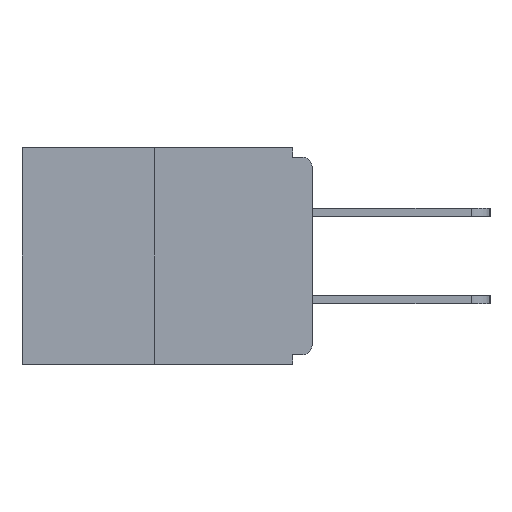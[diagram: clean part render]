
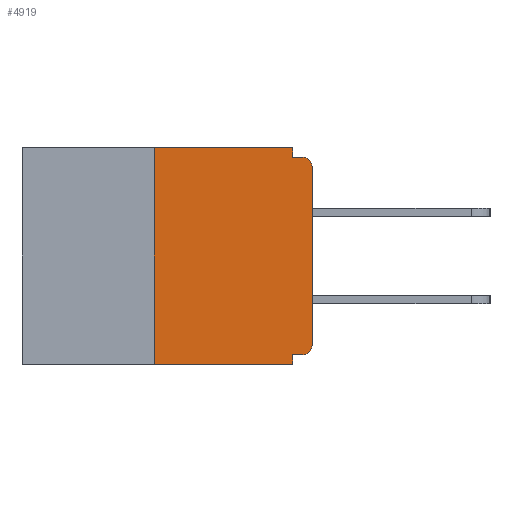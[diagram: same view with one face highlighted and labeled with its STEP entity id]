
A CAD part, left-side view. The second image highlights one B-rep face of the part: STEP entity #4919.
In plain terms, the highlighted planar face has unit normal (-1, 0, 0).
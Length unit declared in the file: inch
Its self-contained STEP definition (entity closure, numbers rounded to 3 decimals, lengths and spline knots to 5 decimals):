
#71 = DIRECTION ( 'NONE',  ( 0., 0., 1. ) ) ;
#465 = VECTOR ( 'NONE', #11201, 39.37008 ) ;
#682 = ORIENTED_EDGE ( 'NONE', *, *, #8445, .F. ) ;
#795 = EDGE_CURVE ( 'NONE', #11745, #6879, #1094, .T. ) ;
#845 = FACE_OUTER_BOUND ( 'NONE', #6350, .T. ) ;
#900 = CARTESIAN_POINT ( 'NONE',  ( 0., 0.25, 0. ) ) ;
#918 = CARTESIAN_POINT ( 'NONE',  ( 0., 0.031, -0.015 ) ) ;
#971 = CARTESIAN_POINT ( 'NONE',  ( 0., 0.25, 0. ) ) ;
#1028 = CARTESIAN_POINT ( 'NONE',  ( 0., 0.46, -0.343 ) ) ;
#1060 = CARTESIAN_POINT ( 'NONE',  ( 0., 0., -0.313 ) ) ;
#1094 = LINE ( 'NONE', #4861, #9689 ) ;
#1195 = EDGE_CURVE ( 'NONE', #1671, #11745, #11263, .T. ) ;
#1282 = AXIS2_PLACEMENT_3D ( 'NONE', #11019, #3575, #7242 ) ;
#1609 = LINE ( 'NONE', #9250, #11494 ) ;
#1671 = VERTEX_POINT ( 'NONE', #9463 ) ;
#1817 = CARTESIAN_POINT ( 'NONE',  ( 0., 0.46, 0. ) ) ;
#2178 = EDGE_CURVE ( 'NONE', #5679, #11479, #9388, .T. ) ;
#2274 = AXIS2_PLACEMENT_3D ( 'NONE', #6519, #6356, #4466 ) ;
#2526 = VERTEX_POINT ( 'NONE', #6142 ) ;
#2614 = VERTEX_POINT ( 'NONE', #918 ) ;
#2723 = ORIENTED_EDGE ( 'NONE', *, *, #6912, .T. ) ;
#2957 = ORIENTED_EDGE ( 'NONE', *, *, #3427, .F. ) ;
#3118 = DIRECTION ( 'NONE',  ( 0., -1., 0. ) ) ;
#3427 = EDGE_CURVE ( 'NONE', #11101, #5679, #6107, .T. ) ;
#3575 = DIRECTION ( 'NONE',  ( -1., 0., 0. ) ) ;
#3594 = ORIENTED_EDGE ( 'NONE', *, *, #4666, .T. ) ;
#3714 = DIRECTION ( 'NONE',  ( 0., 0., -1. ) ) ;
#3778 = VERTEX_POINT ( 'NONE', #9064 ) ;
#3984 = VECTOR ( 'NONE', #3118, 39.37008 ) ;
#4041 = LINE ( 'NONE', #1028, #3984 ) ;
#4174 = CARTESIAN_POINT ( 'NONE',  ( 0., 0.031, -0.343 ) ) ;
#4297 = CARTESIAN_POINT ( 'NONE',  ( 0., 0., -0.328 ) ) ;
#4466 = DIRECTION ( 'NONE',  ( 0., 0., -1. ) ) ;
#4479 = CIRCLE ( 'NONE', #2274, 0.015 ) ;
#4496 = EDGE_CURVE ( 'NONE', #2614, #2526, #9310, .T. ) ;
#4666 = EDGE_CURVE ( 'NONE', #10458, #3778, #7603, .T. ) ;
#4812 = VECTOR ( 'NONE', #8550, 39.37008 ) ;
#4861 = CARTESIAN_POINT ( 'NONE',  ( 0., 0.46, 0. ) ) ;
#4919 = ADVANCED_FACE ( 'NONE', ( #845 ), #8303, .F. ) ;
#4942 = ORIENTED_EDGE ( 'NONE', *, *, #2178, .F. ) ;
#5195 = DIRECTION ( 'NONE',  ( 0., 0., -1. ) ) ;
#5679 = VERTEX_POINT ( 'NONE', #11996 ) ;
#5929 = VECTOR ( 'NONE', #71, 39.37008 ) ;
#6107 = LINE ( 'NONE', #4297, #9466 ) ;
#6142 = CARTESIAN_POINT ( 'NONE',  ( 0., 0.015, -0.015 ) ) ;
#6230 = EDGE_CURVE ( 'NONE', #1671, #11479, #4041, .T. ) ;
#6350 = EDGE_LOOP ( 'NONE', ( #6984, #10186, #9036, #4942, #2957, #7260, #3594, #2723, #8424, #682 ) ) ;
#6356 = DIRECTION ( 'NONE',  ( -1., 0., 0. ) ) ;
#6420 = DIRECTION ( 'NONE',  ( 1., 0., 0. ) ) ;
#6519 = CARTESIAN_POINT ( 'NONE',  ( 0., 0.015, -0.03 ) ) ;
#6621 = CIRCLE ( 'NONE', #1282, 0.015 ) ;
#6879 = VERTEX_POINT ( 'NONE', #9213 ) ;
#6912 = EDGE_CURVE ( 'NONE', #3778, #2526, #4479, .T. ) ;
#6984 = ORIENTED_EDGE ( 'NONE', *, *, #795, .F. ) ;
#7242 = DIRECTION ( 'NONE',  ( 0., 0., -1. ) ) ;
#7260 = ORIENTED_EDGE ( 'NONE', *, *, #11131, .T. ) ;
#7345 = VECTOR ( 'NONE', #3714, 39.37008 ) ;
#7511 = CARTESIAN_POINT ( 'NONE',  ( 0., 0.031, -0.343 ) ) ;
#7603 = LINE ( 'NONE', #7664, #4812 ) ;
#7664 = CARTESIAN_POINT ( 'NONE',  ( 0., 0., 0. ) ) ;
#8303 = PLANE ( 'NONE',  #12193 ) ;
#8424 = ORIENTED_EDGE ( 'NONE', *, *, #4496, .F. ) ;
#8445 = EDGE_CURVE ( 'NONE', #6879, #2614, #1609, .T. ) ;
#8550 = DIRECTION ( 'NONE',  ( 0., 0., 1. ) ) ;
#8675 = DIRECTION ( 'NONE',  ( 0., -1., 0. ) ) ;
#9036 = ORIENTED_EDGE ( 'NONE', *, *, #6230, .T. ) ;
#9064 = CARTESIAN_POINT ( 'NONE',  ( 0., 0., -0.03 ) ) ;
#9213 = CARTESIAN_POINT ( 'NONE',  ( 0., 0.031, 0. ) ) ;
#9250 = CARTESIAN_POINT ( 'NONE',  ( 0., 0.031, 0. ) ) ;
#9310 = LINE ( 'NONE', #11020, #465 ) ;
#9388 = LINE ( 'NONE', #7511, #7345 ) ;
#9463 = CARTESIAN_POINT ( 'NONE',  ( 0., 0.25, -0.343 ) ) ;
#9466 = VECTOR ( 'NONE', #9830, 39.37008 ) ;
#9689 = VECTOR ( 'NONE', #8675, 39.37008 ) ;
#9830 = DIRECTION ( 'NONE',  ( 0., 1., 0. ) ) ;
#9979 = CARTESIAN_POINT ( 'NONE',  ( 0., 0.015, -0.328 ) ) ;
#10186 = ORIENTED_EDGE ( 'NONE', *, *, #1195, .F. ) ;
#10458 = VERTEX_POINT ( 'NONE', #1060 ) ;
#11019 = CARTESIAN_POINT ( 'NONE',  ( 0., 0.015, -0.313 ) ) ;
#11020 = CARTESIAN_POINT ( 'NONE',  ( 0., 0., -0.015 ) ) ;
#11101 = VERTEX_POINT ( 'NONE', #9979 ) ;
#11131 = EDGE_CURVE ( 'NONE', #11101, #10458, #6621, .T. ) ;
#11136 = DIRECTION ( 'NONE',  ( 0., 0., -1. ) ) ;
#11201 = DIRECTION ( 'NONE',  ( 0., -1., 0. ) ) ;
#11263 = LINE ( 'NONE', #971, #5929 ) ;
#11479 = VERTEX_POINT ( 'NONE', #4174 ) ;
#11494 = VECTOR ( 'NONE', #5195, 39.37008 ) ;
#11745 = VERTEX_POINT ( 'NONE', #900 ) ;
#11996 = CARTESIAN_POINT ( 'NONE',  ( 0., 0.031, -0.328 ) ) ;
#12193 = AXIS2_PLACEMENT_3D ( 'NONE', #1817, #6420, #11136 ) ;
